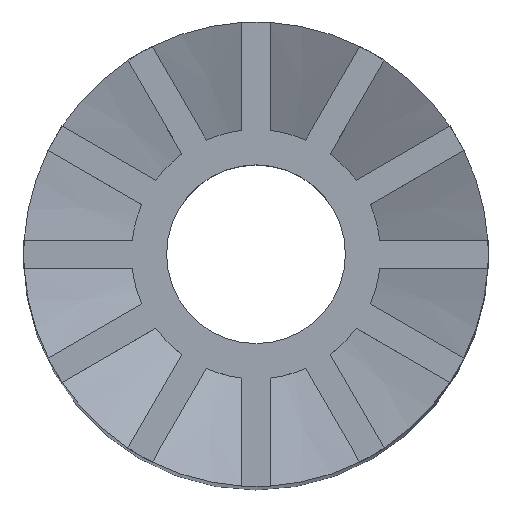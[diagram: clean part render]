
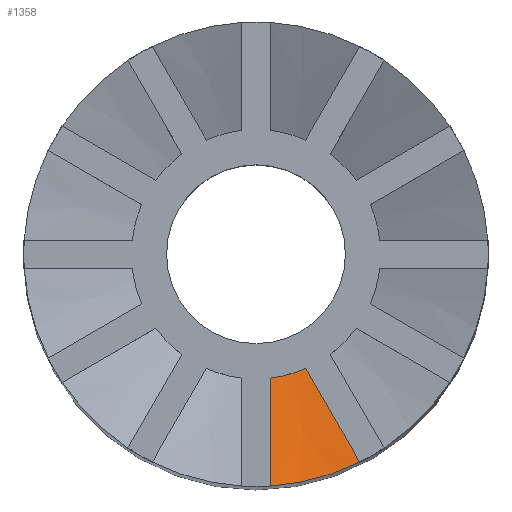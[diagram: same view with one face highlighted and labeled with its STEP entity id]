
A CAD part, top view. The second image highlights one B-rep face of the part: STEP entity #1358.
In plain terms, the highlighted conical face has half-angle 68.587 degrees and reference radius 16.5 mm.
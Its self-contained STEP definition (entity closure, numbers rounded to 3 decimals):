
#1 = AXIS2_PLACEMENT_3D ( 'NONE', #2850, #917, #661 ) ;
#4 = CARTESIAN_POINT ( 'NONE',  ( 1., -16.47, 10. ) ) ;
#62 = B_SPLINE_CURVE_WITH_KNOTS ( 'NONE', 3,
 ( #1282, #796, #1980, #1764 ),
 .UNSPECIFIED., .F., .F.,
 ( 4, 4 ),
 ( 0.01, 0.019 ),
 .UNSPECIFIED. ) ;
#409 = CARTESIAN_POINT ( 'NONE',  ( 4.811, -10.332, 7.997 ) ) ;
#465 = CARTESIAN_POINT ( 'NONE',  ( 3.531, -8.115, 7. ) ) ;
#537 = AXIS2_PLACEMENT_3D ( 'NONE', #1480, #1769, #562 ) ;
#545 = EDGE_CURVE ( 'NONE', #2324, #1569, #2220, .T. ) ;
#561 = ORIENTED_EDGE ( 'NONE', *, *, #2570, .F. ) ;
#562 = DIRECTION ( 'NONE',  ( 1., 0., 0. ) ) ;
#661 = DIRECTION ( 'NONE',  ( 1., 0., 0. ) ) ;
#686 = ORIENTED_EDGE ( 'NONE', *, *, #2865, .T. ) ;
#796 = CARTESIAN_POINT ( 'NONE',  ( 1., -11.353, 7.997 ) ) ;
#917 = DIRECTION ( 'NONE',  ( 0., 0., 1. ) ) ;
#928 = DIRECTION ( 'NONE',  ( 1., 0., 0. ) ) ;
#1229 = VERTEX_POINT ( 'NONE', #2057 ) ;
#1282 = CARTESIAN_POINT ( 'NONE',  ( 1., -8.793, 7. ) ) ;
#1354 = CIRCLE ( 'NONE', #1, 8.85 ) ;
#1358 = ADVANCED_FACE ( 'NONE', ( #2966 ), #2018, .F. ) ;
#1456 = B_SPLINE_CURVE_WITH_KNOTS ( 'NONE', 3,
 ( #1629, #409, #2589, #2316 ),
 .UNSPECIFIED., .F., .F.,
 ( 4, 4 ),
 ( 0., 0.008 ),
 .UNSPECIFIED. ) ;
#1480 = CARTESIAN_POINT ( 'NONE',  ( 0., 0., 10. ) ) ;
#1543 = VERTEX_POINT ( 'NONE', #465 ) ;
#1569 = VERTEX_POINT ( 'NONE', #2635 ) ;
#1629 = CARTESIAN_POINT ( 'NONE',  ( 3.531, -8.115, 7. ) ) ;
#1657 = AXIS2_PLACEMENT_3D ( 'NONE', #2179, #2669, #928 ) ;
#1764 = CARTESIAN_POINT ( 'NONE',  ( 1., -16.47, 10. ) ) ;
#1769 = DIRECTION ( 'NONE',  ( 0., 0., 1. ) ) ;
#1942 = ORIENTED_EDGE ( 'NONE', *, *, #545, .T. ) ;
#1980 = CARTESIAN_POINT ( 'NONE',  ( 1., -13.911, 8.999 ) ) ;
#2018 = CONICAL_SURFACE ( 'NONE', #537, 16.5, 1.197 ) ;
#2057 = CARTESIAN_POINT ( 'NONE',  ( 1., -8.793, 7. ) ) ;
#2179 = CARTESIAN_POINT ( 'NONE',  ( 0., 0., 10. ) ) ;
#2220 = CIRCLE ( 'NONE', #1657, 16.5 ) ;
#2235 = EDGE_CURVE ( 'NONE', #1229, #1543, #1354, .T. ) ;
#2316 = CARTESIAN_POINT ( 'NONE',  ( 7.369, -14.763, 10. ) ) ;
#2324 = VERTEX_POINT ( 'NONE', #4 ) ;
#2570 = EDGE_CURVE ( 'NONE', #1543, #1569, #1456, .T. ) ;
#2589 = CARTESIAN_POINT ( 'NONE',  ( 6.09, -12.548, 8.999 ) ) ;
#2635 = CARTESIAN_POINT ( 'NONE',  ( 7.369, -14.763, 10. ) ) ;
#2669 = DIRECTION ( 'NONE',  ( 0., 0., 1. ) ) ;
#2788 = EDGE_LOOP ( 'NONE', ( #561, #3081, #686, #1942 ) ) ;
#2850 = CARTESIAN_POINT ( 'NONE',  ( 0., 0., 7. ) ) ;
#2865 = EDGE_CURVE ( 'NONE', #1229, #2324, #62, .T. ) ;
#2966 = FACE_OUTER_BOUND ( 'NONE', #2788, .T. ) ;
#3081 = ORIENTED_EDGE ( 'NONE', *, *, #2235, .F. ) ;
